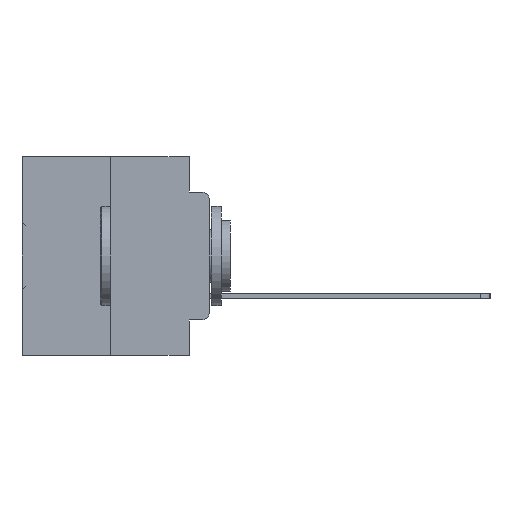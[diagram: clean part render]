
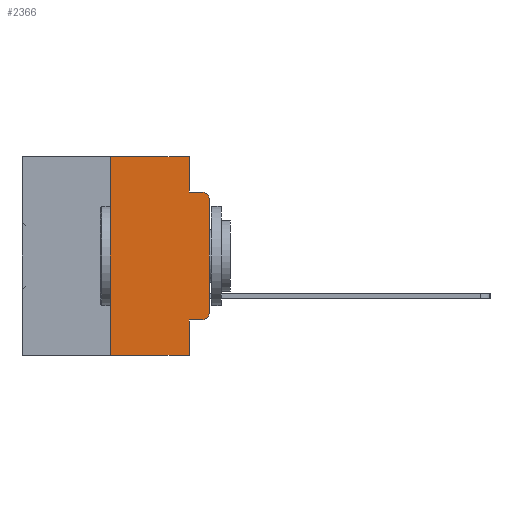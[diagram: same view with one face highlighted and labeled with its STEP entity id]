
A CAD part, left-side view. The second image highlights one B-rep face of the part: STEP entity #2366.
In plain terms, the highlighted planar face has unit normal (-1, 0, 0).
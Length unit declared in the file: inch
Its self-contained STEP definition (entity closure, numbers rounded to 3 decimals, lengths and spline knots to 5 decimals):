
#439 = LINE ( 'NONE', #13447, #7918 ) ;
#1280 = CARTESIAN_POINT ( 'NONE',  ( 0., 0.473, -0.5 ) ) ;
#1909 = VECTOR ( 'NONE', #34085, 39.37008 ) ;
#2294 = LINE ( 'NONE', #5354, #23789 ) ;
#2366 = ADVANCED_FACE ( 'NONE', ( #12378 ), #33804, .F. ) ;
#2771 = VECTOR ( 'NONE', #23708, 39.37008 ) ;
#2982 = AXIS2_PLACEMENT_3D ( 'NONE', #17195, #20039, #3220 ) ;
#3220 = DIRECTION ( 'NONE',  ( 0., 0., -1. ) ) ;
#4108 = DIRECTION ( 'NONE',  ( 0., 0., 1. ) ) ;
#4224 = CIRCLE ( 'NONE', #16840, 0.02 ) ;
#4508 = LINE ( 'NONE', #1280, #2771 ) ;
#4603 = ORIENTED_EDGE ( 'NONE', *, *, #17641, .T. ) ;
#4711 = CARTESIAN_POINT ( 'NONE',  ( 0., 0.02, -0.0885 ) ) ;
#4770 = VECTOR ( 'NONE', #20613, 39.37008 ) ;
#5233 = CARTESIAN_POINT ( 'NONE',  ( 0., 0.02, -0.1085 ) ) ;
#5354 = CARTESIAN_POINT ( 'NONE',  ( 0., 0.051, -0.4115 ) ) ;
#6360 = EDGE_LOOP ( 'NONE', ( #10764, #12532, #19992, #6784, #14294, #8582, #25251, #26112, #4603, #20444 ) ) ;
#6784 = ORIENTED_EDGE ( 'NONE', *, *, #25180, .F. ) ;
#7762 = CARTESIAN_POINT ( 'NONE',  ( 0., 0.051, 0. ) ) ;
#7918 = VECTOR ( 'NONE', #30156, 39.37008 ) ;
#8105 = DIRECTION ( 'NONE',  ( 0., 0., -1. ) ) ;
#8582 = ORIENTED_EDGE ( 'NONE', *, *, #21436, .F. ) ;
#9517 = CARTESIAN_POINT ( 'NONE',  ( 0., 0.051, -0.0885 ) ) ;
#10594 = CARTESIAN_POINT ( 'NONE',  ( 0., 0.02, -0.4115 ) ) ;
#10764 = ORIENTED_EDGE ( 'NONE', *, *, #34366, .T. ) ;
#12026 = EDGE_CURVE ( 'NONE', #23950, #17267, #4224, .T. ) ;
#12378 = FACE_OUTER_BOUND ( 'NONE', #6360, .T. ) ;
#12532 = ORIENTED_EDGE ( 'NONE', *, *, #30720, .T. ) ;
#12848 = CARTESIAN_POINT ( 'NONE',  ( 0., 0.02, -0.3915 ) ) ;
#13169 = LINE ( 'NONE', #34347, #4770 ) ;
#13447 = CARTESIAN_POINT ( 'NONE',  ( 0., 0., 0. ) ) ;
#13872 = DIRECTION ( 'NONE',  ( 0., -1., 0. ) ) ;
#14294 = ORIENTED_EDGE ( 'NONE', *, *, #23558, .F. ) ;
#14620 = VERTEX_POINT ( 'NONE', #7762 ) ;
#14710 = CARTESIAN_POINT ( 'NONE',  ( 0., 0.051, -0.0885 ) ) ;
#15108 = CARTESIAN_POINT ( 'NONE',  ( 0., 0., -0.3915 ) ) ;
#15657 = DIRECTION ( 'NONE',  ( 0., 0., -1. ) ) ;
#16840 = AXIS2_PLACEMENT_3D ( 'NONE', #12848, #32311, #15657 ) ;
#17195 = CARTESIAN_POINT ( 'NONE',  ( 0., 0.473, 0. ) ) ;
#17267 = VERTEX_POINT ( 'NONE', #15108 ) ;
#17281 = LINE ( 'NONE', #28225, #31196 ) ;
#17641 = EDGE_CURVE ( 'NONE', #25061, #23950, #2294, .T. ) ;
#18006 = VERTEX_POINT ( 'NONE', #4711 ) ;
#18621 = CARTESIAN_POINT ( 'NONE',  ( 0., 0.051, -0.4115 ) ) ;
#18854 = VECTOR ( 'NONE', #19108, 39.37008 ) ;
#19108 = DIRECTION ( 'NONE',  ( 0., 0., -1. ) ) ;
#19563 = EDGE_CURVE ( 'NONE', #25061, #28914, #13169, .T. ) ;
#19992 = ORIENTED_EDGE ( 'NONE', *, *, #28885, .F. ) ;
#20039 = DIRECTION ( 'NONE',  ( 1., 0., 0. ) ) ;
#20444 = ORIENTED_EDGE ( 'NONE', *, *, #12026, .T. ) ;
#20509 = CARTESIAN_POINT ( 'NONE',  ( 0., 0., -0.1085 ) ) ;
#20613 = DIRECTION ( 'NONE',  ( 0., 0., -1. ) ) ;
#20769 = VERTEX_POINT ( 'NONE', #23408 ) ;
#21436 = EDGE_CURVE ( 'NONE', #20769, #31525, #24923, .T. ) ;
#23408 = CARTESIAN_POINT ( 'NONE',  ( 0., 0.25, -0.5 ) ) ;
#23558 = EDGE_CURVE ( 'NONE', #31525, #14620, #17281, .T. ) ;
#23708 = DIRECTION ( 'NONE',  ( 0., -1., 0. ) ) ;
#23724 = VERTEX_POINT ( 'NONE', #9517 ) ;
#23773 = EDGE_CURVE ( 'NONE', #20769, #28914, #4508, .T. ) ;
#23789 = VECTOR ( 'NONE', #13872, 39.37008 ) ;
#23950 = VERTEX_POINT ( 'NONE', #10594 ) ;
#24018 = VECTOR ( 'NONE', #4108, 39.37008 ) ;
#24279 = VERTEX_POINT ( 'NONE', #20509 ) ;
#24605 = CARTESIAN_POINT ( 'NONE',  ( 0., 0.051, 0. ) ) ;
#24690 = AXIS2_PLACEMENT_3D ( 'NONE', #5233, #24902, #8105 ) ;
#24902 = DIRECTION ( 'NONE',  ( -1., 0., 0. ) ) ;
#24923 = LINE ( 'NONE', #34679, #24018 ) ;
#25061 = VERTEX_POINT ( 'NONE', #18621 ) ;
#25180 = EDGE_CURVE ( 'NONE', #14620, #23724, #26278, .T. ) ;
#25251 = ORIENTED_EDGE ( 'NONE', *, *, #23773, .T. ) ;
#25946 = CARTESIAN_POINT ( 'NONE',  ( 0., 0.051, -0.5 ) ) ;
#26112 = ORIENTED_EDGE ( 'NONE', *, *, #19563, .F. ) ;
#26278 = LINE ( 'NONE', #24605, #18854 ) ;
#28225 = CARTESIAN_POINT ( 'NONE',  ( 0., 0.473, 0. ) ) ;
#28885 = EDGE_CURVE ( 'NONE', #23724, #18006, #30768, .T. ) ;
#28914 = VERTEX_POINT ( 'NONE', #25946 ) ;
#28956 = CARTESIAN_POINT ( 'NONE',  ( 0., 0.25, 0. ) ) ;
#30156 = DIRECTION ( 'NONE',  ( 0., 0., 1. ) ) ;
#30720 = EDGE_CURVE ( 'NONE', #24279, #18006, #35306, .T. ) ;
#30768 = LINE ( 'NONE', #14710, #1909 ) ;
#31196 = VECTOR ( 'NONE', #33704, 39.37008 ) ;
#31525 = VERTEX_POINT ( 'NONE', #28956 ) ;
#32311 = DIRECTION ( 'NONE',  ( -1., 0., 0. ) ) ;
#33704 = DIRECTION ( 'NONE',  ( 0., -1., 0. ) ) ;
#33804 = PLANE ( 'NONE',  #2982 ) ;
#34085 = DIRECTION ( 'NONE',  ( 0., -1., 0. ) ) ;
#34347 = CARTESIAN_POINT ( 'NONE',  ( 0., 0.051, 0. ) ) ;
#34366 = EDGE_CURVE ( 'NONE', #17267, #24279, #439, .T. ) ;
#34679 = CARTESIAN_POINT ( 'NONE',  ( 0., 0.25, 0. ) ) ;
#35306 = CIRCLE ( 'NONE', #24690, 0.02 ) ;
